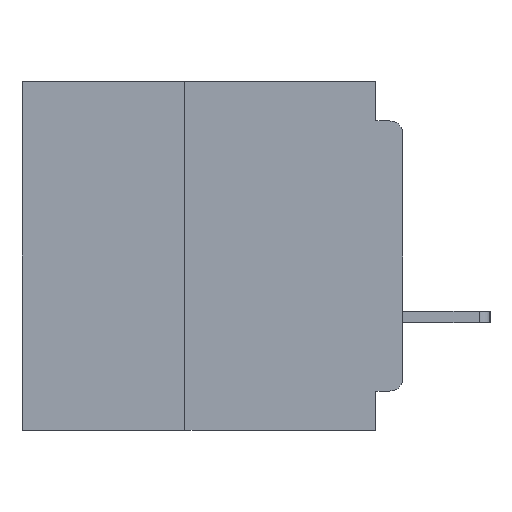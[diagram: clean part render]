
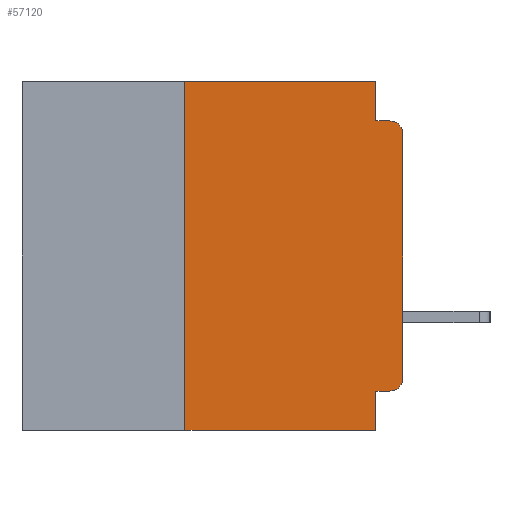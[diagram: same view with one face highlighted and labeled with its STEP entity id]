
A CAD part, left-side view. The second image highlights one B-rep face of the part: STEP entity #57120.
In plain terms, the highlighted planar face has unit normal (-1, 0, 0).
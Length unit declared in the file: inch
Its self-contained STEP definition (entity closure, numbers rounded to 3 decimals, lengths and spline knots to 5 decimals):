
#76 = AXIS2_PLACEMENT_3D ( 'NONE', #14987, #59820, #30059 ) ;
#661 = EDGE_CURVE ( 'NONE', #15521, #44529, #28109, .T. ) ;
#2760 = CARTESIAN_POINT ( 'NONE',  ( 0., 0.015, -0.045 ) ) ;
#3781 = DIRECTION ( 'NONE',  ( 0., 0., -1. ) ) ;
#6306 = ORIENTED_EDGE ( 'NONE', *, *, #55644, .F. ) ;
#6474 = ORIENTED_EDGE ( 'NONE', *, *, #24065, .F. ) ;
#6860 = AXIS2_PLACEMENT_3D ( 'NONE', #8009, #42971, #13039 ) ;
#6961 = VECTOR ( 'NONE', #3781, 39.37008 ) ;
#7545 = VERTEX_POINT ( 'NONE', #35644 ) ;
#8009 = CARTESIAN_POINT ( 'NONE',  ( 0., 0.015, -0.06 ) ) ;
#8514 = LINE ( 'NONE', #63640, #6961 ) ;
#9432 = VECTOR ( 'NONE', #24458, 39.37008 ) ;
#9639 = CARTESIAN_POINT ( 'NONE',  ( 0., 0.437, 0. ) ) ;
#10070 = CARTESIAN_POINT ( 'NONE',  ( 0., 0.031, -0.045 ) ) ;
#11400 = CARTESIAN_POINT ( 'NONE',  ( 0., 0., -0.06 ) ) ;
#11945 = CARTESIAN_POINT ( 'NONE',  ( 0., 0.031, -0.4 ) ) ;
#12014 = EDGE_CURVE ( 'NONE', #7545, #44928, #13967, .T. ) ;
#12083 = VERTEX_POINT ( 'NONE', #10070 ) ;
#12594 = EDGE_CURVE ( 'NONE', #22633, #29806, #39692, .T. ) ;
#13039 = DIRECTION ( 'NONE',  ( 0., 0., -1. ) ) ;
#13278 = DIRECTION ( 'NONE',  ( 0., 0., -1. ) ) ;
#13483 = DIRECTION ( 'NONE',  ( -1., 0., 0. ) ) ;
#13967 = LINE ( 'NONE', #9639, #38979 ) ;
#14000 = EDGE_CURVE ( 'NONE', #61930, #29806, #35682, .T. ) ;
#14987 = CARTESIAN_POINT ( 'NONE',  ( 0., 0.437, 0. ) ) ;
#15521 = VERTEX_POINT ( 'NONE', #48060 ) ;
#15783 = CARTESIAN_POINT ( 'NONE',  ( 0., 0.25, -0.4 ) ) ;
#15882 = CARTESIAN_POINT ( 'NONE',  ( 0., 0., -0.355 ) ) ;
#18365 = AXIS2_PLACEMENT_3D ( 'NONE', #63986, #13483, #13278 ) ;
#19293 = ORIENTED_EDGE ( 'NONE', *, *, #14000, .F. ) ;
#19696 = DIRECTION ( 'NONE',  ( 0., -1., 0. ) ) ;
#19833 = LINE ( 'NONE', #15882, #44866 ) ;
#20081 = CARTESIAN_POINT ( 'NONE',  ( 0., 0.437, -0.4 ) ) ;
#21160 = ORIENTED_EDGE ( 'NONE', *, *, #12594, .T. ) ;
#22633 = VERTEX_POINT ( 'NONE', #15783 ) ;
#23503 = EDGE_CURVE ( 'NONE', #51611, #28978, #42354, .T. ) ;
#24065 = EDGE_CURVE ( 'NONE', #12083, #28978, #34432, .T. ) ;
#24335 = VECTOR ( 'NONE', #53925, 39.37008 ) ;
#24458 = DIRECTION ( 'NONE',  ( 0., -1., 0. ) ) ;
#24747 = EDGE_CURVE ( 'NONE', #15521, #61930, #19833, .T. ) ;
#26446 = VECTOR ( 'NONE', #30118, 39.37008 ) ;
#28109 = CIRCLE ( 'NONE', #18365, 0.015 ) ;
#28978 = VERTEX_POINT ( 'NONE', #2760 ) ;
#29806 = VERTEX_POINT ( 'NONE', #60530 ) ;
#30059 = DIRECTION ( 'NONE',  ( 0., 0., -1. ) ) ;
#30118 = DIRECTION ( 'NONE',  ( 0., -1., 0. ) ) ;
#30331 = VECTOR ( 'NONE', #36250, 39.37008 ) ;
#31242 = CARTESIAN_POINT ( 'NONE',  ( 0., 0., 0. ) ) ;
#33434 = FACE_OUTER_BOUND ( 'NONE', #42412, .T. ) ;
#34432 = LINE ( 'NONE', #59243, #9432 ) ;
#35644 = CARTESIAN_POINT ( 'NONE',  ( 0., 0.25, 0. ) ) ;
#35682 = LINE ( 'NONE', #11945, #58964 ) ;
#35738 = DIRECTION ( 'NONE',  ( 0., 1., 0. ) ) ;
#36070 = CARTESIAN_POINT ( 'NONE',  ( 0., 0., -0.34 ) ) ;
#36250 = DIRECTION ( 'NONE',  ( 0., 0., 1. ) ) ;
#37049 = DIRECTION ( 'NONE',  ( 0., 0., -1. ) ) ;
#38979 = VECTOR ( 'NONE', #19696, 39.37008 ) ;
#39692 = LINE ( 'NONE', #20081, #26446 ) ;
#40030 = ORIENTED_EDGE ( 'NONE', *, *, #12014, .F. ) ;
#40510 = EDGE_CURVE ( 'NONE', #44529, #51611, #58332, .T. ) ;
#41326 = ORIENTED_EDGE ( 'NONE', *, *, #23503, .T. ) ;
#42354 = CIRCLE ( 'NONE', #6860, 0.015 ) ;
#42412 = EDGE_LOOP ( 'NONE', ( #47754, #41326, #6474, #6306, #40030, #52545, #21160, #19293, #53319, #54937 ) ) ;
#42971 = DIRECTION ( 'NONE',  ( -1., 0., 0. ) ) ;
#44529 = VERTEX_POINT ( 'NONE', #36070 ) ;
#44866 = VECTOR ( 'NONE', #35738, 39.37008 ) ;
#44928 = VERTEX_POINT ( 'NONE', #49276 ) ;
#47754 = ORIENTED_EDGE ( 'NONE', *, *, #40510, .T. ) ;
#48060 = CARTESIAN_POINT ( 'NONE',  ( 0., 0.015, -0.355 ) ) ;
#48950 = CARTESIAN_POINT ( 'NONE',  ( 0., 0.25, -0.4 ) ) ;
#49276 = CARTESIAN_POINT ( 'NONE',  ( 0., 0.031, 0. ) ) ;
#50844 = LINE ( 'NONE', #48950, #24335 ) ;
#51307 = EDGE_CURVE ( 'NONE', #22633, #7545, #50844, .T. ) ;
#51611 = VERTEX_POINT ( 'NONE', #11400 ) ;
#52545 = ORIENTED_EDGE ( 'NONE', *, *, #51307, .F. ) ;
#53319 = ORIENTED_EDGE ( 'NONE', *, *, #24747, .F. ) ;
#53925 = DIRECTION ( 'NONE',  ( 0., 0., 1. ) ) ;
#54874 = PLANE ( 'NONE',  #76 ) ;
#54937 = ORIENTED_EDGE ( 'NONE', *, *, #661, .T. ) ;
#55644 = EDGE_CURVE ( 'NONE', #44928, #12083, #8514, .T. ) ;
#57120 = ADVANCED_FACE ( 'NONE', ( #33434 ), #54874, .F. ) ;
#58332 = LINE ( 'NONE', #31242, #30331 ) ;
#58964 = VECTOR ( 'NONE', #37049, 39.37008 ) ;
#59243 = CARTESIAN_POINT ( 'NONE',  ( 0., 0., -0.045 ) ) ;
#59820 = DIRECTION ( 'NONE',  ( 1., 0., 0. ) ) ;
#60530 = CARTESIAN_POINT ( 'NONE',  ( 0., 0.031, -0.4 ) ) ;
#61930 = VERTEX_POINT ( 'NONE', #64374 ) ;
#63640 = CARTESIAN_POINT ( 'NONE',  ( 0., 0.031, 0. ) ) ;
#63986 = CARTESIAN_POINT ( 'NONE',  ( 0., 0.015, -0.34 ) ) ;
#64374 = CARTESIAN_POINT ( 'NONE',  ( 0., 0.031, -0.355 ) ) ;
